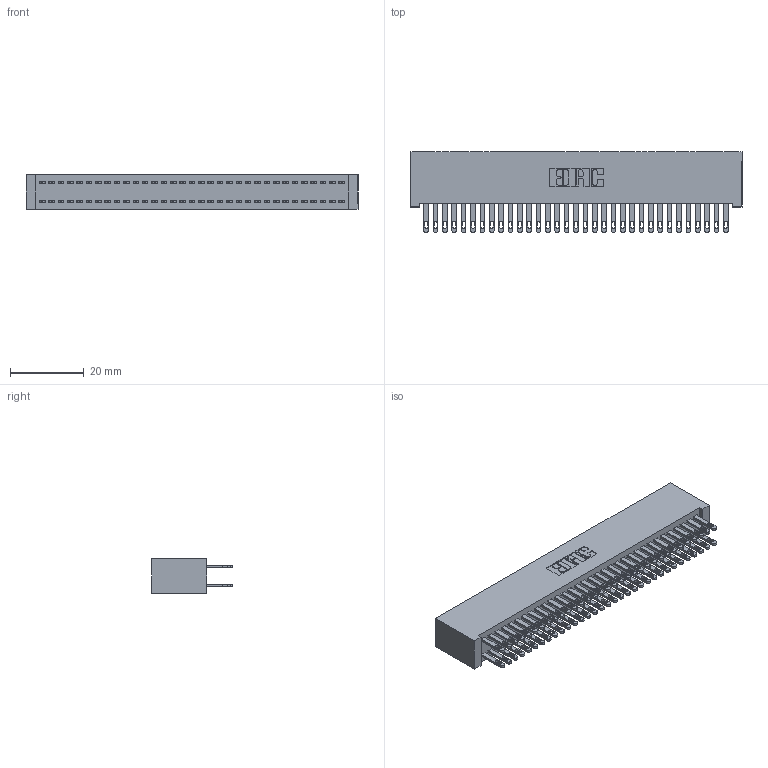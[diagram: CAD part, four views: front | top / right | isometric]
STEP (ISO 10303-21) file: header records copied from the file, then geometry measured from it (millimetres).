
FILE_DESCRIPTION (( 'STEP AP203' ), '1' );
FILE_NAME ('342-066-500-201.STEP', '2018-08-13T07:45:14', ( '' ), ( '' ), 'SwSTEP 2.0', 'SolidWorks 2016', '' );
FILE_SCHEMA (( 'CONFIG_CONTROL_DESIGN' ));
Length unit declared in the file: inch
Products named in the file (3): 345-292-001_345-293-100; 342-066-500-201; 342 Part_Lugless
Assembly tree (67 placements, depth 2):
  342-066-500-201
    342 Part_Lugless
    345-292-001_345-293-100  x66
Bounding box: 90.07 x 21.85 x 9.4 mm (x, y, z)
Volume: 8691.2 mm3; surface area: 15003.5 mm2
Topology: 67 solids, 67 shells, 3270 faces, 9977 edges, 6650 vertices
Faces by surface type: plane 2042, cylinder 1228
Entity records: 21915 total; most frequent: CARTESIAN_POINT 3638, ORIENTED_EDGE 3574, DIRECTION 3119, EDGE_CURVE 1787, VECTOR 1663, LINE 1663, VERTEX_POINT 1190, AXIS2_PLACEMENT_3D 728
